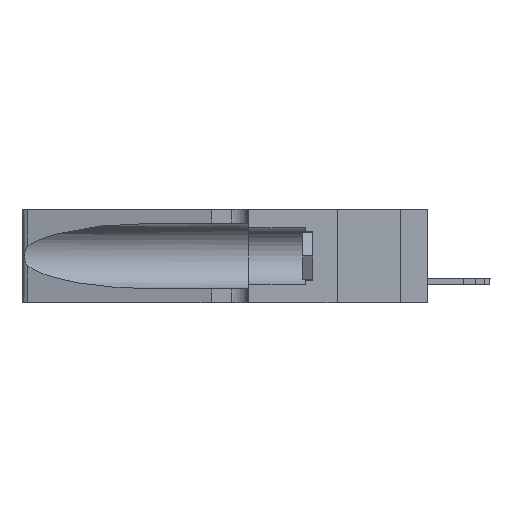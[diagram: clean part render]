
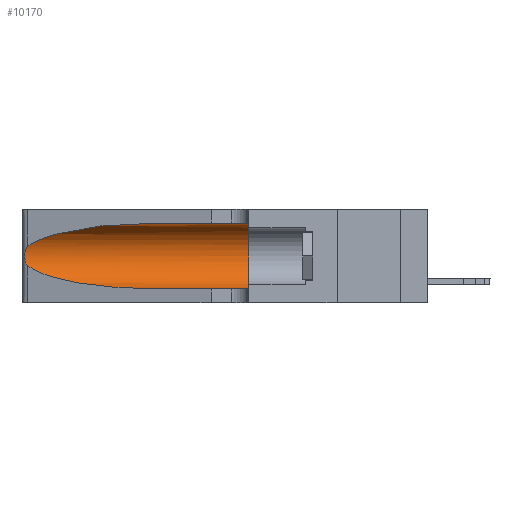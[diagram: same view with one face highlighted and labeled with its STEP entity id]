
A CAD part, left-side view. The second image highlights one B-rep face of the part: STEP entity #10170.
In plain terms, the highlighted cylindrical face has radius 3.308 mm (diameter 6.617 mm), a partial arc.
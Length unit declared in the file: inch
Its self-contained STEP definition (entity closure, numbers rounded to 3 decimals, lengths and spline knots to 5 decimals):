
#346 = CYLINDRICAL_SURFACE ( 'NONE', #6105, 0.13025 ) ;
#1187 = EDGE_CURVE ( 'NONE', #2025, #6385, #18082, .T. ) ;
#1274 = CARTESIAN_POINT ( 'NONE',  ( 0.1305, 0.35, 0.185 ) ) ;
#1344 = DIRECTION ( 'NONE',  ( 0., 1., 0. ) ) ;
#1612 = CARTESIAN_POINT ( 'NONE',  ( 0.26075, 1.23896, 0.178 ) ) ;
#1792 = VERTEX_POINT ( 'NONE', #18204 ) ;
#1915 =( BOUNDED_CURVE ( )  B_SPLINE_CURVE ( 3, ( #17797, #10130, #5606, #10263 ),
 .UNSPECIFIED., .F., .F. ) 
 B_SPLINE_CURVE_WITH_KNOTS ( ( 4, 4 ),
 ( 1.5708, 2.84003 ),
 .UNSPECIFIED. ) 
 CURVE ( )  GEOMETRIC_REPRESENTATION_ITEM ( )  RATIONAL_B_SPLINE_CURVE ( ( 1., 0.87, 0.87, 1. ) ) 
 REPRESENTATION_ITEM ( '' )  );
#2025 = VERTEX_POINT ( 'NONE', #17123 ) ;
#2814 = DIRECTION ( 'NONE',  ( 0., -1., 0. ) ) ;
#2849 = CARTESIAN_POINT ( 'NONE',  ( 0.26075, 1.23896, 0.19203 ) ) ;
#2935 = LINE ( 'NONE', #2945, #4116 ) ;
#2945 = CARTESIAN_POINT ( 'NONE',  ( 0.1305, 1.61858, 0.31525 ) ) ;
#2981 = CARTESIAN_POINT ( 'NONE',  ( 0.25555, 1.22994, 0.2215 ) ) ;
#3441 = EDGE_CURVE ( 'NONE', #8686, #14711, #14118, .T. ) ;
#3568 = CARTESIAN_POINT ( 'NONE',  ( 0.1305, 0.72297, 0.05475 ) ) ;
#3867 = AXIS2_PLACEMENT_3D ( 'NONE', #1274, #1344, #5620 ) ;
#4116 = VECTOR ( 'NONE', #2814, 39.37008 ) ;
#4207 = DIRECTION ( 'NONE',  ( 0., -1., 0. ) ) ;
#4684 = LINE ( 'NONE', #11275, #17708 ) ;
#5606 = CARTESIAN_POINT ( 'NONE',  ( 0.2373, 1.15595, 0.28018 ) ) ;
#5620 = DIRECTION ( 'NONE',  ( 0., 0., 1. ) ) ;
#6043 = B_SPLINE_CURVE_WITH_KNOTS ( 'NONE', 3,
 ( #9171, #2981, #6170, #19477, #12097, #13612, #2849, #1612, #15008, #18225, #15071, #18032, #19616, #7699 ),
 .UNSPECIFIED., .F., .F.,
 ( 4, 2, 2, 2, 2, 2, 4 ),
 ( 0., 0.00027, 0.00053, 0.00107, 0.0016, 0.00187, 0.00214 ),
 .UNSPECIFIED. ) ;
#6105 = AXIS2_PLACEMENT_3D ( 'NONE', #7384, #4207, #10444 ) ;
#6170 = CARTESIAN_POINT ( 'NONE',  ( 0.25639, 1.23184, 0.21858 ) ) ;
#6385 = VERTEX_POINT ( 'NONE', #3568 ) ;
#6858 = CARTESIAN_POINT ( 'NONE',  ( 0.18966, 0.96281, 0.05475 ) ) ;
#6986 = CARTESIAN_POINT ( 'NONE',  ( 0.1305, 0.35, 0.05475 ) ) ;
#7384 = CARTESIAN_POINT ( 'NONE',  ( 0.1305, 1.61858, 0.185 ) ) ;
#7699 = CARTESIAN_POINT ( 'NONE',  ( 0.25487, 1.22718, 0.14631 ) ) ;
#7916 = EDGE_CURVE ( 'NONE', #6385, #14711, #4684, .T. ) ;
#7919 = ORIENTED_EDGE ( 'NONE', *, *, #15470, .T. ) ;
#8205 = CARTESIAN_POINT ( 'NONE',  ( 0.25487, 1.22718, 0.14631 ) ) ;
#8686 = VERTEX_POINT ( 'NONE', #16829 ) ;
#9171 = CARTESIAN_POINT ( 'NONE',  ( 0.25487, 1.22718, 0.22369 ) ) ;
#9552 = EDGE_CURVE ( 'NONE', #17980, #1792, #1915, .T. ) ;
#10130 = CARTESIAN_POINT ( 'NONE',  ( 0.18966, 0.96281, 0.31525 ) ) ;
#10170 = ADVANCED_FACE ( 'NONE', ( #14101 ), #346, .F. ) ;
#10263 = CARTESIAN_POINT ( 'NONE',  ( 0.25487, 1.22718, 0.22369 ) ) ;
#10442 = ORIENTED_EDGE ( 'NONE', *, *, #1187, .T. ) ;
#10444 = DIRECTION ( 'NONE',  ( 0., 0., -1. ) ) ;
#10931 = CARTESIAN_POINT ( 'NONE',  ( 0.1305, 0.72297, 0.31525 ) ) ;
#11275 = CARTESIAN_POINT ( 'NONE',  ( 0.1305, 1.61858, 0.05475 ) ) ;
#12097 = CARTESIAN_POINT ( 'NONE',  ( 0.25854, 1.2359, 0.20912 ) ) ;
#12777 = CARTESIAN_POINT ( 'NONE',  ( 0.2373, 1.15595, 0.08982 ) ) ;
#12807 = DIRECTION ( 'NONE',  ( 0., -1., 0. ) ) ;
#13156 = ORIENTED_EDGE ( 'NONE', *, *, #7916, .T. ) ;
#13219 = ORIENTED_EDGE ( 'NONE', *, *, #16509, .F. ) ;
#13612 = CARTESIAN_POINT ( 'NONE',  ( 0.26018, 1.23835, 0.19895 ) ) ;
#14101 = FACE_OUTER_BOUND ( 'NONE', #17225, .T. ) ;
#14118 = CIRCLE ( 'NONE', #3867, 0.13025 ) ;
#14311 = CARTESIAN_POINT ( 'NONE',  ( 0.1305, 0.72297, 0.05475 ) ) ;
#14711 = VERTEX_POINT ( 'NONE', #6986 ) ;
#15008 = CARTESIAN_POINT ( 'NONE',  ( 0.26017, 1.23833, 0.17102 ) ) ;
#15071 = CARTESIAN_POINT ( 'NONE',  ( 0.25789, 1.23486, 0.15765 ) ) ;
#15336 = ORIENTED_EDGE ( 'NONE', *, *, #9552, .T. ) ;
#15470 = EDGE_CURVE ( 'NONE', #1792, #2025, #6043, .T. ) ;
#16509 = EDGE_CURVE ( 'NONE', #17980, #8686, #2935, .T. ) ;
#16829 = CARTESIAN_POINT ( 'NONE',  ( 0.1305, 0.35, 0.31525 ) ) ;
#17123 = CARTESIAN_POINT ( 'NONE',  ( 0.25487, 1.22718, 0.14631 ) ) ;
#17225 = EDGE_LOOP ( 'NONE', ( #15336, #7919, #10442, #13156, #17811, #13219 ) ) ;
#17708 = VECTOR ( 'NONE', #12807, 39.37008 ) ;
#17797 = CARTESIAN_POINT ( 'NONE',  ( 0.1305, 0.72297, 0.31525 ) ) ;
#17811 = ORIENTED_EDGE ( 'NONE', *, *, #3441, .F. ) ;
#17980 = VERTEX_POINT ( 'NONE', #10931 ) ;
#18032 = CARTESIAN_POINT ( 'NONE',  ( 0.25639, 1.23186, 0.15144 ) ) ;
#18082 =( BOUNDED_CURVE ( )  B_SPLINE_CURVE ( 3, ( #8205, #12777, #6858, #14311 ),
 .UNSPECIFIED., .F., .F. ) 
 B_SPLINE_CURVE_WITH_KNOTS ( ( 4, 4 ),
 ( 3.44316, 4.71239 ),
 .UNSPECIFIED. ) 
 CURVE ( )  GEOMETRIC_REPRESENTATION_ITEM ( )  RATIONAL_B_SPLINE_CURVE ( ( 1., 0.87, 0.87, 1. ) ) 
 REPRESENTATION_ITEM ( '' )  );
#18204 = CARTESIAN_POINT ( 'NONE',  ( 0.25487, 1.22718, 0.22369 ) ) ;
#18225 = CARTESIAN_POINT ( 'NONE',  ( 0.25856, 1.23593, 0.16098 ) ) ;
#19477 = CARTESIAN_POINT ( 'NONE',  ( 0.25787, 1.23484, 0.2124 ) ) ;
#19616 = CARTESIAN_POINT ( 'NONE',  ( 0.25555, 1.22993, 0.14849 ) ) ;
